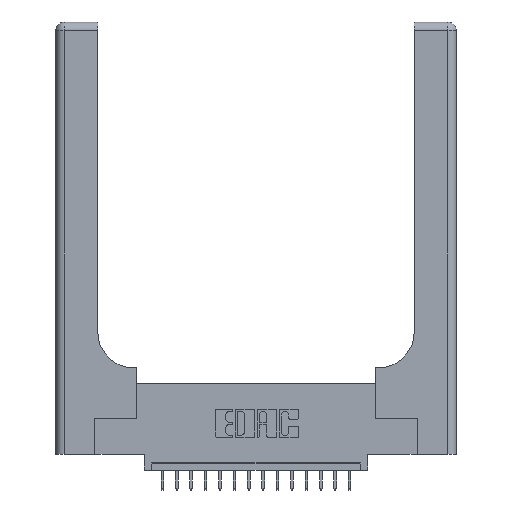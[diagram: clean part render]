
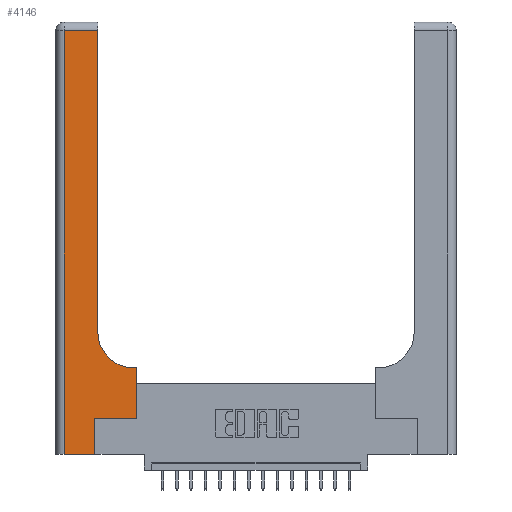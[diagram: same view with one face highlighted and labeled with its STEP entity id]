
A CAD part, top view. The second image highlights one B-rep face of the part: STEP entity #4146.
In plain terms, the highlighted planar face has unit normal (0, 0, 1).
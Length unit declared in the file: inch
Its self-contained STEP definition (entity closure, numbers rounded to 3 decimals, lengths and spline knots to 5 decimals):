
#120 = ORIENTED_EDGE ( 'NONE', *, *, #3660, .T. ) ;
#311 = CARTESIAN_POINT ( 'NONE',  ( 0.269, 0.25, 0.37 ) ) ;
#348 = ORIENTED_EDGE ( 'NONE', *, *, #12249, .T. ) ;
#793 = CARTESIAN_POINT ( 'NONE',  ( 0.2915, 0.6, 0.37 ) ) ;
#1121 = ORIENTED_EDGE ( 'NONE', *, *, #5148, .T. ) ;
#1178 = DIRECTION ( 'NONE',  ( 0., -1., 0. ) ) ;
#1244 = VERTEX_POINT ( 'NONE', #9954 ) ;
#1307 = DIRECTION ( 'NONE',  ( -1., 0., 0. ) ) ;
#1705 = AXIS2_PLACEMENT_3D ( 'NONE', #15340, #12063, #18264 ) ;
#1752 = VERTEX_POINT ( 'NONE', #10794 ) ;
#2241 = EDGE_CURVE ( 'NONE', #7108, #19139, #3567, .T. ) ;
#2605 = CARTESIAN_POINT ( 'NONE',  ( 0.269, 0., 0.37 ) ) ;
#3168 = DIRECTION ( 'NONE',  ( 0., 0., -1. ) ) ;
#3217 = VERTEX_POINT ( 'NONE', #9801 ) ;
#3258 = EDGE_LOOP ( 'NONE', ( #15896, #17540, #3326, #1121, #120, #18053, #16866, #13835, #348 ) ) ;
#3300 = DIRECTION ( 'NONE',  ( 0., 1., 0. ) ) ;
#3326 = ORIENTED_EDGE ( 'NONE', *, *, #11181, .T. ) ;
#3567 = LINE ( 'NONE', #311, #13797 ) ;
#3660 = EDGE_CURVE ( 'NONE', #6000, #7108, #11499, .T. ) ;
#4146 = ADVANCED_FACE ( 'NONE', ( #4668 ), #4465, .F. ) ;
#4392 = VERTEX_POINT ( 'NONE', #19622 ) ;
#4465 = PLANE ( 'NONE',  #9337 ) ;
#4668 = FACE_OUTER_BOUND ( 'NONE', #3258, .T. ) ;
#4762 = EDGE_CURVE ( 'NONE', #14848, #4392, #8001, .T. ) ;
#4969 = VECTOR ( 'NONE', #10568, 39.37008 ) ;
#5148 = EDGE_CURVE ( 'NONE', #1244, #6000, #14632, .T. ) ;
#5562 = CARTESIAN_POINT ( 'NONE',  ( 0., 0., 0.37 ) ) ;
#5568 = CARTESIAN_POINT ( 'NONE',  ( 0.06, 3., 0.37 ) ) ;
#6000 = VERTEX_POINT ( 'NONE', #2605 ) ;
#6960 = CARTESIAN_POINT ( 'NONE',  ( 0., 2.94, 0.37 ) ) ;
#7090 = VECTOR ( 'NONE', #11615, 39.37008 ) ;
#7108 = VERTEX_POINT ( 'NONE', #17899 ) ;
#7450 = VERTEX_POINT ( 'NONE', #11880 ) ;
#8001 = LINE ( 'NONE', #17011, #11547 ) ;
#9101 = LINE ( 'NONE', #12073, #4969 ) ;
#9337 = AXIS2_PLACEMENT_3D ( 'NONE', #10775, #3168, #1307 ) ;
#9638 = VECTOR ( 'NONE', #14726, 39.37008 ) ;
#9801 = CARTESIAN_POINT ( 'NONE',  ( 0.5585, 0.6, 0.37 ) ) ;
#9954 = CARTESIAN_POINT ( 'NONE',  ( 0.06, 0., 0.37 ) ) ;
#10568 = DIRECTION ( 'NONE',  ( 0., 1., 0. ) ) ;
#10775 = CARTESIAN_POINT ( 'NONE',  ( 0., 3., 0.37 ) ) ;
#10794 = CARTESIAN_POINT ( 'NONE',  ( 0.06, 2.94, 0.37 ) ) ;
#10982 = LINE ( 'NONE', #793, #19567 ) ;
#11024 = EDGE_CURVE ( 'NONE', #3217, #7450, #10982, .T. ) ;
#11181 = EDGE_CURVE ( 'NONE', #1752, #1244, #18135, .T. ) ;
#11469 = LINE ( 'NONE', #6960, #18725 ) ;
#11499 = LINE ( 'NONE', #17606, #7090 ) ;
#11547 = VECTOR ( 'NONE', #3300, 39.37008 ) ;
#11615 = DIRECTION ( 'NONE',  ( 0., 1., 0. ) ) ;
#11880 = CARTESIAN_POINT ( 'NONE',  ( 0.5415, 0.6, 0.37 ) ) ;
#12063 = DIRECTION ( 'NONE',  ( 0., 0., -1. ) ) ;
#12073 = CARTESIAN_POINT ( 'NONE',  ( 0.5585, 0.25, 0.37 ) ) ;
#12249 = EDGE_CURVE ( 'NONE', #7450, #14848, #14762, .T. ) ;
#13071 = DIRECTION ( 'NONE',  ( -1., 0., 0. ) ) ;
#13797 = VECTOR ( 'NONE', #13898, 39.37008 ) ;
#13835 = ORIENTED_EDGE ( 'NONE', *, *, #11024, .T. ) ;
#13898 = DIRECTION ( 'NONE',  ( 1., 0., 0. ) ) ;
#14167 = CARTESIAN_POINT ( 'NONE',  ( 0.2915, 0.85, 0.37 ) ) ;
#14632 = LINE ( 'NONE', #5562, #9638 ) ;
#14726 = DIRECTION ( 'NONE',  ( 1., 0., 0. ) ) ;
#14762 = CIRCLE ( 'NONE', #1705, 0.25 ) ;
#14848 = VERTEX_POINT ( 'NONE', #14167 ) ;
#15340 = CARTESIAN_POINT ( 'NONE',  ( 0.5415, 0.85, 0.37 ) ) ;
#15896 = ORIENTED_EDGE ( 'NONE', *, *, #4762, .T. ) ;
#16040 = CARTESIAN_POINT ( 'NONE',  ( 0.5585, 0.25, 0.37 ) ) ;
#16046 = EDGE_CURVE ( 'NONE', #19139, #3217, #9101, .T. ) ;
#16866 = ORIENTED_EDGE ( 'NONE', *, *, #16046, .T. ) ;
#17011 = CARTESIAN_POINT ( 'NONE',  ( 0.2915, 3., 0.37 ) ) ;
#17540 = ORIENTED_EDGE ( 'NONE', *, *, #18801, .T. ) ;
#17606 = CARTESIAN_POINT ( 'NONE',  ( 0.269, 0., 0.37 ) ) ;
#17899 = CARTESIAN_POINT ( 'NONE',  ( 0.269, 0.25, 0.37 ) ) ;
#17944 = VECTOR ( 'NONE', #1178, 39.37008 ) ;
#18053 = ORIENTED_EDGE ( 'NONE', *, *, #2241, .T. ) ;
#18135 = LINE ( 'NONE', #5568, #17944 ) ;
#18264 = DIRECTION ( 'NONE',  ( 1., 0., 0. ) ) ;
#18725 = VECTOR ( 'NONE', #13071, 39.37008 ) ;
#18755 = DIRECTION ( 'NONE',  ( -1., 0., 0. ) ) ;
#18801 = EDGE_CURVE ( 'NONE', #4392, #1752, #11469, .T. ) ;
#19139 = VERTEX_POINT ( 'NONE', #16040 ) ;
#19567 = VECTOR ( 'NONE', #18755, 39.37008 ) ;
#19622 = CARTESIAN_POINT ( 'NONE',  ( 0.2915, 2.94, 0.37 ) ) ;
